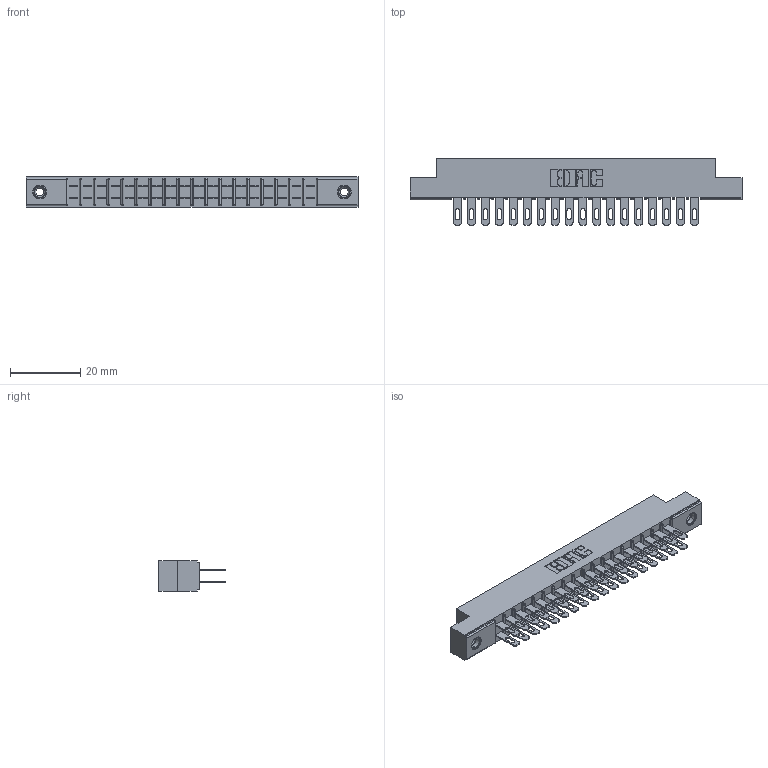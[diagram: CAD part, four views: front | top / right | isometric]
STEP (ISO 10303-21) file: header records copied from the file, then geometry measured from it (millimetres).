
FILE_DESCRIPTION (( 'STEP AP203' ), '1' );
FILE_NAME ('315-036-500-208.STEP', '2019-09-10T16:05:32', ( '' ), ( '' ), 'SwSTEP 2.0', 'SolidWorks 2016', '' );
FILE_SCHEMA (( 'CONFIG_CONTROL_DESIGN' ));
Length unit declared in the file: inch
Products named in the file (4): 315-036-500-208; 305-290-001_500; 345-250-001_345-250-003-102; 305 Part_.156 Dia
Assembly tree (39 placements, depth 2):
  315-036-500-208
    305 Part_.156 Dia
    305-290-001_500  x36
    345-250-001_345-250-003-102  x2
Bounding box: 94.34 x 18.85 x 8.71 mm (x, y, z)
Volume: 6031.2 mm3; surface area: 11800 mm2
Topology: 39 solids, 39 shells, 1976 faces, 5618 edges, 3640 vertices
Faces by surface type: plane 1108, cylinder 780, sphere 72, cone 12, torus 4
Entity records: 23618 total; most frequent: CARTESIAN_POINT 3891, ORIENTED_EDGE 3852, DIRECTION 3796, EDGE_CURVE 1926, VECTOR 1526, LINE 1526, VERTEX_POINT 1230, AXIS2_PLACEMENT_3D 1135
